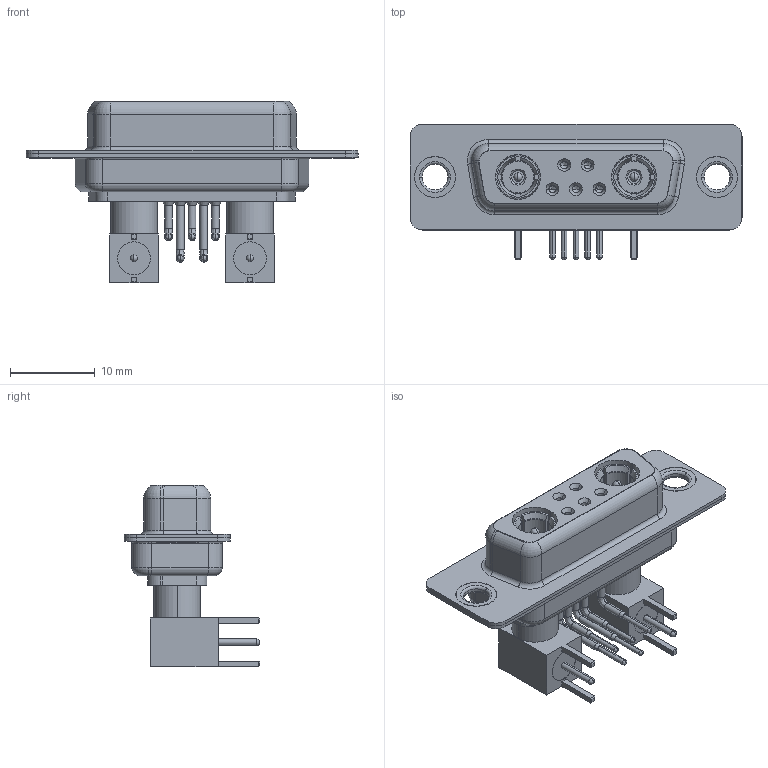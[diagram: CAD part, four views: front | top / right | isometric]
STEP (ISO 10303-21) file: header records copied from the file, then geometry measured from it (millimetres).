
FILE_DESCRIPTION (( 'STEP AP203' ), '1' );
FILE_NAME ('630-7W2-640-5N1.STEP', '2022-05-31T05:09:12', ( '' ), ( '' ), 'SwSTEP 2.0', 'SolidWorks 2020', '' );
FILE_SCHEMA (( 'CONFIG_CONTROL_DESIGN' ));
Length unit declared in the file: millimetre
Products named in the file (15): 630Combo Housing_7W2; Insulator RA Pin; Insulator Pin_Straight PC Tail; 630Combo Shell Front_15 Contacts; Co-Ax Plug Assy_RA; Locking Collar; 630Combo Contact Row 2; 630Combo Contact Row 1; 630Combo Thru Hole Rivet; 630-7W2-640-5N1; RA Back Shell; Pin_RA; Co-Ax Plug_RA PC Tail; 630Combo Shell Rear_15 Contacts
Assembly tree (24 placements, depth 3):
  630-7W2-640-5N1
    630Combo Housing_7W2
    630Combo Shell Front_15 Contacts
    630Combo Shell Rear_15 Contacts
    630Combo Thru Hole Rivet  x2
    Co-Ax Plug Assy_RA
      Co-Ax Plug_RA PC Tail
      Insulator Pin_Straight PC Tail
      Pin_RA
      Locking Collar
      RA Back Shell
      Insulator RA Pin
    Co-Ax Plug Assy_RA
      Co-Ax Plug_RA PC Tail
      Insulator Pin_Straight PC Tail
      Pin_RA
      Locking Collar
      RA Back Shell
      Insulator RA Pin
    630Combo Contact Row 1  x2
    630Combo Contact Row 2  x3
Bounding box: 39.2 x 16 x 21.41 mm (x, y, z)
Volume: 2895.9 mm3; surface area: 7180.4 mm2
Topology: 22 solids, 22 shells, 854 faces, 2080 edges, 1298 vertices
Faces by surface type: cylinder 366, plane 276, cone 105, torus 77, bspline 22, sphere 8
Entity records: 18440 total; most frequent: CARTESIAN_POINT 3315, DIRECTION 3029, ORIENTED_EDGE 2620, EDGE_CURVE 1310, AXIS2_PLACEMENT_3D 1235, VERTEX_POINT 828, CIRCLE 664, EDGE_LOOP 632
